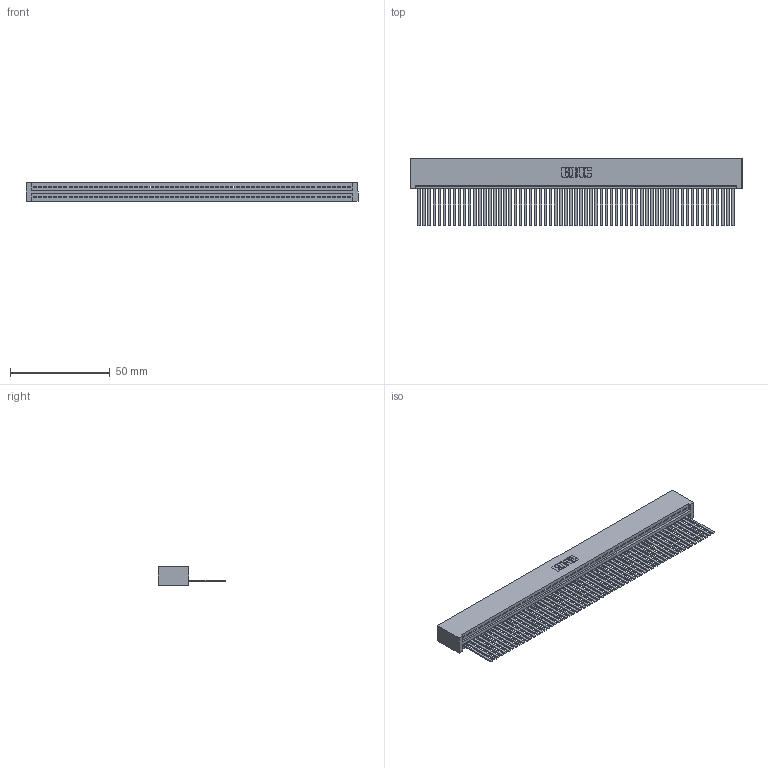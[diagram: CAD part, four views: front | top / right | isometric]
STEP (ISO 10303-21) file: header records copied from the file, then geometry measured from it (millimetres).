
FILE_DESCRIPTION (( 'STEP AP203' ), '1' );
FILE_NAME ('345-063-544-101.STEP', '2019-10-11T11:54:11', ( '' ), ( '' ), 'SwSTEP 2.0', 'SolidWorks 2016', '' );
FILE_SCHEMA (( 'CONFIG_CONTROL_DESIGN' ));
Length unit declared in the file: inch
Products named in the file (3): 345 Part_No Mounting Lugs; 345-063-544-101; 345-292-001_345-293-144
Assembly tree (64 placements, depth 2):
  345-063-544-101
    345 Part_No Mounting Lugs
    345-292-001_345-293-144  x63
Bounding box: 166.62 x 33.96 x 9.4 mm (x, y, z)
Volume: 17312.1 mm3; surface area: 25672.2 mm2
Topology: 64 solids, 64 shells, 3394 faces, 10271 edges, 6762 vertices
Faces by surface type: plane 2344, cylinder 1050
Entity records: 44127 total; most frequent: CARTESIAN_POINT 7649, ORIENTED_EDGE 7646, DIRECTION 6641, EDGE_CURVE 3823, LINE 3451, VECTOR 3451, VERTEX_POINT 2546, AXIS2_PLACEMENT_3D 1595
